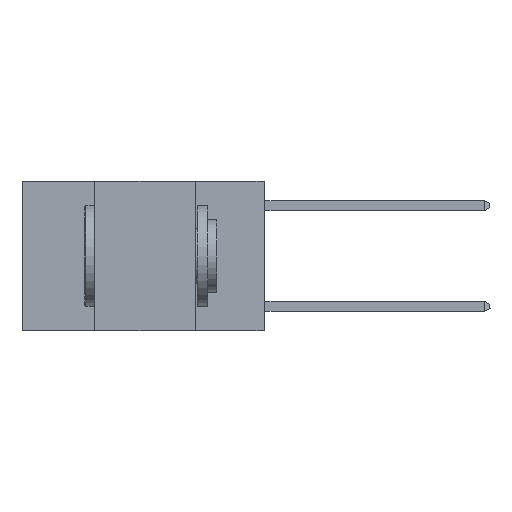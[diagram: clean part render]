
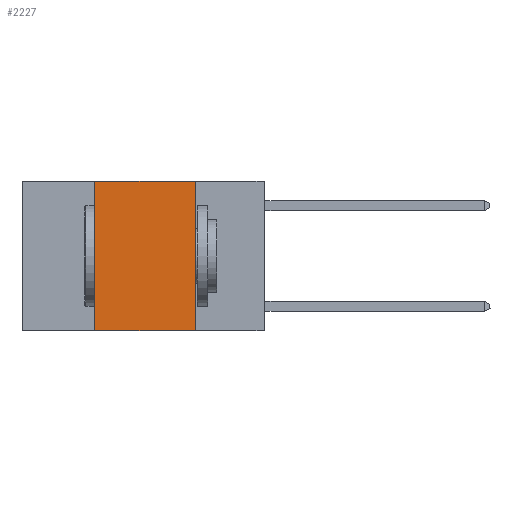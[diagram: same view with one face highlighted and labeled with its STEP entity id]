
A CAD part, left-side view. The second image highlights one B-rep face of the part: STEP entity #2227.
In plain terms, the highlighted planar face has unit normal (-1, 0, 0).
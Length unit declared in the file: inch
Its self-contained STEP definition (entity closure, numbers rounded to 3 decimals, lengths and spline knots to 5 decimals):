
#72 = EDGE_CURVE ( 'NONE', #3090, #10694, #10182, .T. ) ;
#431 = ORIENTED_EDGE ( 'NONE', *, *, #4428, .T. ) ;
#492 = DIRECTION ( 'NONE',  ( 1., 0., 0. ) ) ;
#1032 = LINE ( 'NONE', #8937, #12072 ) ;
#1285 = LINE ( 'NONE', #4014, #12664 ) ;
#1789 = AXIS2_PLACEMENT_3D ( 'NONE', #12606, #492, #2720 ) ;
#2227 = ADVANCED_FACE ( 'NONE', ( #6566 ), #3338, .F. ) ;
#2327 = EDGE_CURVE ( 'NONE', #7388, #3090, #11448, .T. ) ;
#2720 = DIRECTION ( 'NONE',  ( 0., 0., -1. ) ) ;
#3090 = VERTEX_POINT ( 'NONE', #13501 ) ;
#3338 = PLANE ( 'NONE',  #1789 ) ;
#4014 = CARTESIAN_POINT ( 'NONE',  ( 0., 0.42, 0. ) ) ;
#4428 = EDGE_CURVE ( 'NONE', #6480, #10694, #1032, .T. ) ;
#5293 = DIRECTION ( 'NONE',  ( 0., 0., 1. ) ) ;
#5551 = ORIENTED_EDGE ( 'NONE', *, *, #72, .F. ) ;
#6195 = ORIENTED_EDGE ( 'NONE', *, *, #2327, .F. ) ;
#6480 = VERTEX_POINT ( 'NONE', #12355 ) ;
#6566 = FACE_OUTER_BOUND ( 'NONE', #12136, .T. ) ;
#7024 = ORIENTED_EDGE ( 'NONE', *, *, #7698, .F. ) ;
#7185 = VECTOR ( 'NONE', #10652, 39.37008 ) ;
#7388 = VERTEX_POINT ( 'NONE', #10168 ) ;
#7698 = EDGE_CURVE ( 'NONE', #6480, #7388, #1285, .T. ) ;
#8219 = CARTESIAN_POINT ( 'NONE',  ( 0., 0.17, 0. ) ) ;
#8688 = CARTESIAN_POINT ( 'NONE',  ( 0., 0.17, -0.37 ) ) ;
#8937 = CARTESIAN_POINT ( 'NONE',  ( 0., 0.6, -0.37 ) ) ;
#10168 = CARTESIAN_POINT ( 'NONE',  ( 0., 0.42, 0. ) ) ;
#10182 = LINE ( 'NONE', #8219, #7185 ) ;
#10652 = DIRECTION ( 'NONE',  ( 0., 0., -1. ) ) ;
#10694 = VERTEX_POINT ( 'NONE', #8688 ) ;
#10709 = DIRECTION ( 'NONE',  ( 0., -1., 0. ) ) ;
#11112 = VECTOR ( 'NONE', #10709, 39.37008 ) ;
#11448 = LINE ( 'NONE', #12068, #11112 ) ;
#12068 = CARTESIAN_POINT ( 'NONE',  ( 0., 0.6, 0. ) ) ;
#12072 = VECTOR ( 'NONE', #12264, 39.37008 ) ;
#12136 = EDGE_LOOP ( 'NONE', ( #5551, #6195, #7024, #431 ) ) ;
#12264 = DIRECTION ( 'NONE',  ( 0., -1., 0. ) ) ;
#12355 = CARTESIAN_POINT ( 'NONE',  ( 0., 0.42, -0.37 ) ) ;
#12606 = CARTESIAN_POINT ( 'NONE',  ( 0., 0.6, 0. ) ) ;
#12664 = VECTOR ( 'NONE', #5293, 39.37008 ) ;
#13501 = CARTESIAN_POINT ( 'NONE',  ( 0., 0.17, 0. ) ) ;
